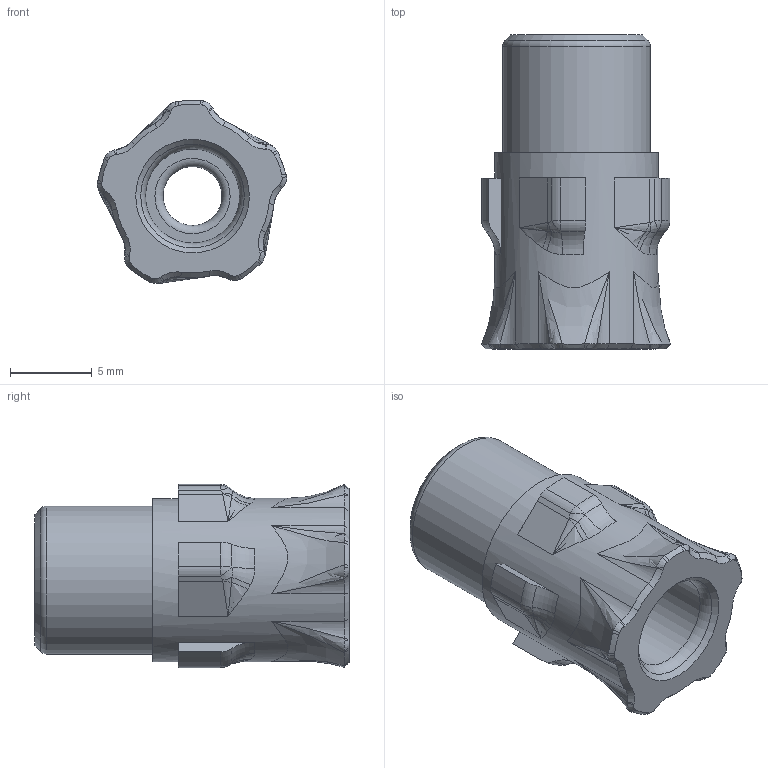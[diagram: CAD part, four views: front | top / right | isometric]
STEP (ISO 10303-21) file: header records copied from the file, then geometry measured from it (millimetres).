
FILE_DESCRIPTION(/* description */ (''),/* implementation_level */ '2;1');
FILE_NAME(/* name */ 'Cartridge Retaining Spindle.step',/* time_stamp */ '2021-05-12T09:10:44-04:00',/* author */ (''),/* organization */ (''),/* preprocessor_version */ 'ST-DEVELOPER v18.1',/* originating_system */ 'Autodesk Translation Framework v10.6.0.1341',/* authorisation */ '');
FILE_SCHEMA (('AUTOMOTIVE_DESIGN { 1 0 10303 214 3 1 1 }'));
Length unit declared in the file: millimetre
Products named in the file (1): Cartridge Retaining Spindle
Bounding box: 11.57 x 19.2 x 11.2 mm (x, y, z)
Volume: 1073.3 mm3; surface area: 1048.1 mm2
Topology: 1 solids, 1 shells, 165 faces, 423 edges, 247 vertices
Faces by surface type: bspline 80, cylinder 24, plane 24, cone 18, torus 14, sphere 5
Full cylindrical faces by diameter (mm): 3.6 x1, 5.75 x1, 9.05 x1, 10 x1
Entity records: 6902 total; most frequent: CARTESIAN_POINT 3494, ORIENTED_EDGE 806, DIRECTION 514, EDGE_CURVE 403, VERTEX_POINT 247, AXIS2_PLACEMENT_3D 201, B_SPLINE_CURVE_WITH_KNOTS 176, EDGE_LOOP 174
